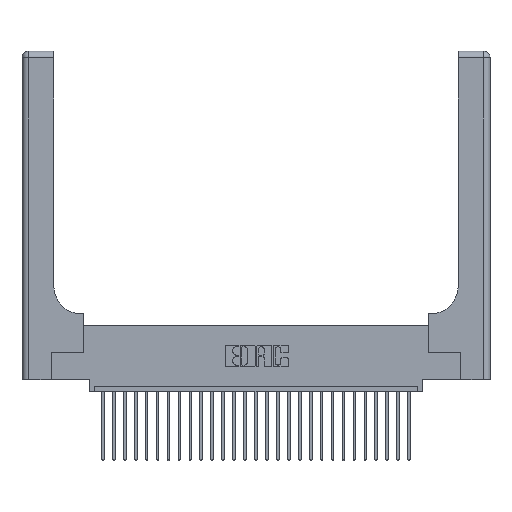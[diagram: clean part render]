
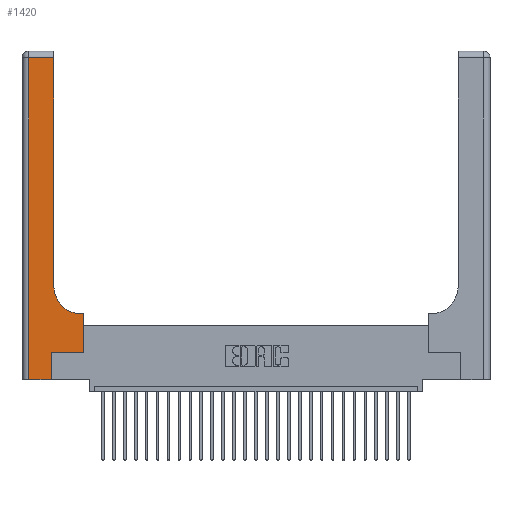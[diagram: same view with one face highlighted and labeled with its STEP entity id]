
A CAD part, top view. The second image highlights one B-rep face of the part: STEP entity #1420.
In plain terms, the highlighted planar face has unit normal (0, 0, 1).
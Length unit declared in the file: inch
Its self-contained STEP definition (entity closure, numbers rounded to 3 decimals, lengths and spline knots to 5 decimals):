
#45 = CARTESIAN_POINT ( 'NONE',  ( 0.269, 0.25, 0.37 ) ) ;
#273 = EDGE_CURVE ( 'NONE', #26220, #1219, #24434, .T. ) ;
#310 = CARTESIAN_POINT ( 'NONE',  ( 0.5415, 0.6, 0.37 ) ) ;
#352 = EDGE_CURVE ( 'NONE', #21129, #6485, #19506, .T. ) ;
#539 = CARTESIAN_POINT ( 'NONE',  ( 0.06, 2.94, 0.37 ) ) ;
#1219 = VERTEX_POINT ( 'NONE', #7364 ) ;
#1349 = CARTESIAN_POINT ( 'NONE',  ( 0.2915, 2.94, 0.37 ) ) ;
#1407 = CARTESIAN_POINT ( 'NONE',  ( 0.5415, 0.85, 0.37 ) ) ;
#1420 = ADVANCED_FACE ( 'NONE', ( #13505 ), #14408, .F. ) ;
#1749 = DIRECTION ( 'NONE',  ( 0., 1., 0. ) ) ;
#2062 = VECTOR ( 'NONE', #5150, 39.37008 ) ;
#3484 = DIRECTION ( 'NONE',  ( 0., 0., -1. ) ) ;
#3832 = DIRECTION ( 'NONE',  ( 1., 0., 0. ) ) ;
#3948 = CARTESIAN_POINT ( 'NONE',  ( 0.5585, 0.25, 0.37 ) ) ;
#4036 = CARTESIAN_POINT ( 'NONE',  ( 0.06, 0., 0.37 ) ) ;
#4236 = DIRECTION ( 'NONE',  ( 0., 0., -1. ) ) ;
#5150 = DIRECTION ( 'NONE',  ( -1., 0., 0. ) ) ;
#5701 = DIRECTION ( 'NONE',  ( 1., 0., 0. ) ) ;
#6007 = ORIENTED_EDGE ( 'NONE', *, *, #8284, .T. ) ;
#6033 = ORIENTED_EDGE ( 'NONE', *, *, #6297, .T. ) ;
#6041 = VECTOR ( 'NONE', #17044, 39.37008 ) ;
#6297 = EDGE_CURVE ( 'NONE', #23397, #26220, #23296, .T. ) ;
#6485 = VERTEX_POINT ( 'NONE', #4036 ) ;
#7224 = CARTESIAN_POINT ( 'NONE',  ( 0.5585, 0.6, 0.37 ) ) ;
#7364 = CARTESIAN_POINT ( 'NONE',  ( 0.2915, 0.85, 0.37 ) ) ;
#7824 = DIRECTION ( 'NONE',  ( -1., 0., 0. ) ) ;
#8284 = EDGE_CURVE ( 'NONE', #6485, #21026, #9469, .T. ) ;
#8634 = CARTESIAN_POINT ( 'NONE',  ( 0.269, 0., 0.37 ) ) ;
#9469 = LINE ( 'NONE', #12595, #14364 ) ;
#9513 = VECTOR ( 'NONE', #21135, 39.37008 ) ;
#11005 = ORIENTED_EDGE ( 'NONE', *, *, #11464, .T. ) ;
#11127 = LINE ( 'NONE', #18439, #2062 ) ;
#11461 = LINE ( 'NONE', #24115, #24736 ) ;
#11464 = EDGE_CURVE ( 'NONE', #28260, #21129, #11127, .T. ) ;
#12595 = CARTESIAN_POINT ( 'NONE',  ( 0., 0., 0.37 ) ) ;
#12636 = EDGE_LOOP ( 'NONE', ( #23062, #11005, #17227, #6007, #13916, #17763, #22886, #6033, #28674 ) ) ;
#13070 = VERTEX_POINT ( 'NONE', #22356 ) ;
#13407 = DIRECTION ( 'NONE',  ( 1., 0., 0. ) ) ;
#13505 = FACE_OUTER_BOUND ( 'NONE', #12636, .T. ) ;
#13916 = ORIENTED_EDGE ( 'NONE', *, *, #28199, .T. ) ;
#14364 = VECTOR ( 'NONE', #3832, 39.37008 ) ;
#14408 = PLANE ( 'NONE',  #21327 ) ;
#15406 = CARTESIAN_POINT ( 'NONE',  ( 0.2915, 0.6, 0.37 ) ) ;
#15832 = CARTESIAN_POINT ( 'NONE',  ( 0.06, 3., 0.37 ) ) ;
#17044 = DIRECTION ( 'NONE',  ( 0., 1., 0. ) ) ;
#17227 = ORIENTED_EDGE ( 'NONE', *, *, #352, .T. ) ;
#17763 = ORIENTED_EDGE ( 'NONE', *, *, #17828, .T. ) ;
#17828 = EDGE_CURVE ( 'NONE', #13070, #20285, #18018, .T. ) ;
#18018 = LINE ( 'NONE', #45, #19404 ) ;
#18083 = VECTOR ( 'NONE', #20353, 39.37008 ) ;
#18251 = EDGE_CURVE ( 'NONE', #20285, #23397, #20694, .T. ) ;
#18439 = CARTESIAN_POINT ( 'NONE',  ( 0., 2.94, 0.37 ) ) ;
#19404 = VECTOR ( 'NONE', #13407, 39.37008 ) ;
#19506 = LINE ( 'NONE', #15832, #18083 ) ;
#19816 = DIRECTION ( 'NONE',  ( -1., 0., 0. ) ) ;
#19968 = LINE ( 'NONE', #21235, #9513 ) ;
#20285 = VERTEX_POINT ( 'NONE', #3948 ) ;
#20353 = DIRECTION ( 'NONE',  ( 0., -1., 0. ) ) ;
#20694 = LINE ( 'NONE', #27961, #6041 ) ;
#21026 = VERTEX_POINT ( 'NONE', #8634 ) ;
#21129 = VERTEX_POINT ( 'NONE', #539 ) ;
#21135 = DIRECTION ( 'NONE',  ( 0., 1., 0. ) ) ;
#21235 = CARTESIAN_POINT ( 'NONE',  ( 0.269, 0., 0.37 ) ) ;
#21327 = AXIS2_PLACEMENT_3D ( 'NONE', #22980, #4236, #7824 ) ;
#22356 = CARTESIAN_POINT ( 'NONE',  ( 0.269, 0.25, 0.37 ) ) ;
#22886 = ORIENTED_EDGE ( 'NONE', *, *, #18251, .T. ) ;
#22980 = CARTESIAN_POINT ( 'NONE',  ( 0., 3., 0.37 ) ) ;
#23062 = ORIENTED_EDGE ( 'NONE', *, *, #25781, .T. ) ;
#23296 = LINE ( 'NONE', #15406, #26083 ) ;
#23397 = VERTEX_POINT ( 'NONE', #7224 ) ;
#23765 = AXIS2_PLACEMENT_3D ( 'NONE', #1407, #3484, #5701 ) ;
#24115 = CARTESIAN_POINT ( 'NONE',  ( 0.2915, 3., 0.37 ) ) ;
#24434 = CIRCLE ( 'NONE', #23765, 0.25 ) ;
#24736 = VECTOR ( 'NONE', #1749, 39.37008 ) ;
#25781 = EDGE_CURVE ( 'NONE', #1219, #28260, #11461, .T. ) ;
#26083 = VECTOR ( 'NONE', #19816, 39.37008 ) ;
#26220 = VERTEX_POINT ( 'NONE', #310 ) ;
#27961 = CARTESIAN_POINT ( 'NONE',  ( 0.5585, 0.25, 0.37 ) ) ;
#28199 = EDGE_CURVE ( 'NONE', #21026, #13070, #19968, .T. ) ;
#28260 = VERTEX_POINT ( 'NONE', #1349 ) ;
#28674 = ORIENTED_EDGE ( 'NONE', *, *, #273, .T. ) ;
